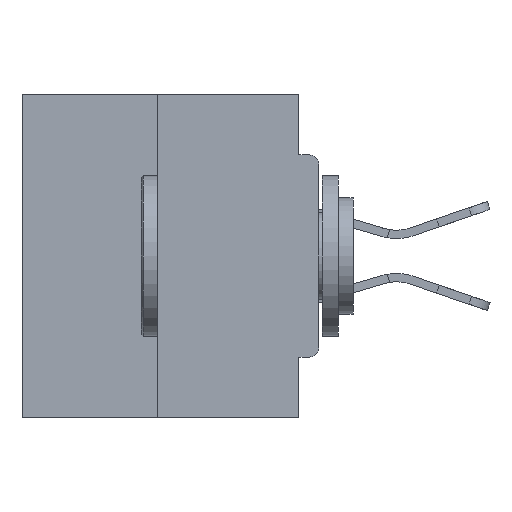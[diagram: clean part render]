
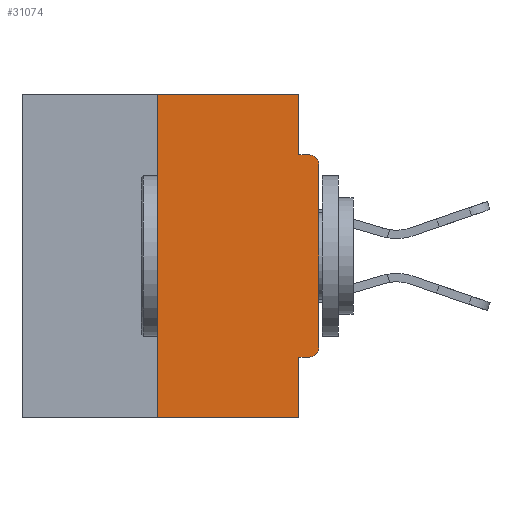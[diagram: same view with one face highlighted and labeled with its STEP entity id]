
A CAD part, left-side view. The second image highlights one B-rep face of the part: STEP entity #31074.
In plain terms, the highlighted planar face has unit normal (-1, 0, 0).
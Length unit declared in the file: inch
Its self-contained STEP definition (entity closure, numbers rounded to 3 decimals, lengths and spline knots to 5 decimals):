
#179 = CARTESIAN_POINT ( 'NONE',  ( 0., 0.25, 0. ) ) ;
#206 = CARTESIAN_POINT ( 'NONE',  ( 0., 0.46, 0. ) ) ;
#354 = VECTOR ( 'NONE', #16216, 39.37008 ) ;
#511 = VECTOR ( 'NONE', #19148, 39.37008 ) ;
#738 = AXIS2_PLACEMENT_3D ( 'NONE', #16466, #16011, #10956 ) ;
#1168 = VERTEX_POINT ( 'NONE', #29994 ) ;
#1659 = CIRCLE ( 'NONE', #30910, 0.015 ) ;
#1946 = CARTESIAN_POINT ( 'NONE',  ( 0., 0.031, 0. ) ) ;
#2277 = ORIENTED_EDGE ( 'NONE', *, *, #3938, .F. ) ;
#2723 = CARTESIAN_POINT ( 'NONE',  ( 0., 0.015, -0.0935 ) ) ;
#3280 = EDGE_CURVE ( 'NONE', #1168, #25429, #1659, .T. ) ;
#3938 = EDGE_CURVE ( 'NONE', #28312, #7588, #29198, .T. ) ;
#5595 = CARTESIAN_POINT ( 'NONE',  ( 0., 0.031, -0.0935 ) ) ;
#6081 = CARTESIAN_POINT ( 'NONE',  ( 0., 0., 0. ) ) ;
#6090 = CARTESIAN_POINT ( 'NONE',  ( 0., 0., -0.3915 ) ) ;
#6240 = VECTOR ( 'NONE', #16872, 39.37008 ) ;
#6244 = EDGE_CURVE ( 'NONE', #25429, #11616, #7592, .T. ) ;
#6886 = DIRECTION ( 'NONE',  ( 0., -1., 0. ) ) ;
#6990 = DIRECTION ( 'NONE',  ( 1., 0., 0. ) ) ;
#7049 = LINE ( 'NONE', #22115, #6240 ) ;
#7381 = CARTESIAN_POINT ( 'NONE',  ( 0., 0.46, -0.5 ) ) ;
#7588 = VERTEX_POINT ( 'NONE', #19410 ) ;
#7592 = LINE ( 'NONE', #6081, #511 ) ;
#8652 = AXIS2_PLACEMENT_3D ( 'NONE', #33786, #6990, #25566 ) ;
#9234 = VECTOR ( 'NONE', #6886, 39.37008 ) ;
#10273 = ORIENTED_EDGE ( 'NONE', *, *, #6244, .T. ) ;
#10285 = CARTESIAN_POINT ( 'NONE',  ( 0., 0.031, -0.5 ) ) ;
#10792 = DIRECTION ( 'NONE',  ( 0., 0., 1. ) ) ;
#10956 = DIRECTION ( 'NONE',  ( 0., 0., -1. ) ) ;
#11283 = LINE ( 'NONE', #7381, #29266 ) ;
#11456 = CARTESIAN_POINT ( 'NONE',  ( 0., 0.031, -0.4065 ) ) ;
#11616 = VERTEX_POINT ( 'NONE', #18738 ) ;
#11720 = ORIENTED_EDGE ( 'NONE', *, *, #3280, .T. ) ;
#12069 = CARTESIAN_POINT ( 'NONE',  ( 0., 0.25, -0.5 ) ) ;
#12322 = VECTOR ( 'NONE', #23061, 39.37008 ) ;
#12788 = DIRECTION ( 'NONE',  ( 0., 1., 0. ) ) ;
#13453 = CARTESIAN_POINT ( 'NONE',  ( 0., 0.015, -0.3915 ) ) ;
#13629 = VERTEX_POINT ( 'NONE', #2723 ) ;
#13695 = DIRECTION ( 'NONE',  ( 0., 0., -1. ) ) ;
#13709 = ORIENTED_EDGE ( 'NONE', *, *, #25088, .F. ) ;
#16011 = DIRECTION ( 'NONE',  ( -1., 0., 0. ) ) ;
#16216 = DIRECTION ( 'NONE',  ( 0., -1., 0. ) ) ;
#16372 = LINE ( 'NONE', #33573, #9234 ) ;
#16466 = CARTESIAN_POINT ( 'NONE',  ( 0., 0.015, -0.1085 ) ) ;
#16708 = EDGE_CURVE ( 'NONE', #1168, #32036, #33486, .T. ) ;
#16737 = ORIENTED_EDGE ( 'NONE', *, *, #19901, .F. ) ;
#16872 = DIRECTION ( 'NONE',  ( 0., 0., -1. ) ) ;
#16969 = EDGE_CURVE ( 'NONE', #32036, #25229, #7049, .T. ) ;
#17366 = ORIENTED_EDGE ( 'NONE', *, *, #26324, .T. ) ;
#17911 = CARTESIAN_POINT ( 'NONE',  ( 0., 0., -0.4065 ) ) ;
#18673 = DIRECTION ( 'NONE',  ( -1., 0., 0. ) ) ;
#18738 = CARTESIAN_POINT ( 'NONE',  ( 0., 0., -0.1085 ) ) ;
#19148 = DIRECTION ( 'NONE',  ( 0., 0., 1. ) ) ;
#19262 = PLANE ( 'NONE',  #8652 ) ;
#19410 = CARTESIAN_POINT ( 'NONE',  ( 0., 0.031, 0. ) ) ;
#19901 = EDGE_CURVE ( 'NONE', #22623, #13629, #16372, .T. ) ;
#21442 = ORIENTED_EDGE ( 'NONE', *, *, #16708, .F. ) ;
#22115 = CARTESIAN_POINT ( 'NONE',  ( 0., 0.031, -0.5 ) ) ;
#22623 = VERTEX_POINT ( 'NONE', #5595 ) ;
#22775 = LINE ( 'NONE', #1946, #12322 ) ;
#23061 = DIRECTION ( 'NONE',  ( 0., 0., -1. ) ) ;
#23544 = CIRCLE ( 'NONE', #738, 0.015 ) ;
#25088 = EDGE_CURVE ( 'NONE', #7588, #22623, #22775, .T. ) ;
#25229 = VERTEX_POINT ( 'NONE', #10285 ) ;
#25429 = VERTEX_POINT ( 'NONE', #6090 ) ;
#25566 = DIRECTION ( 'NONE',  ( 0., 0., -1. ) ) ;
#25662 = CARTESIAN_POINT ( 'NONE',  ( 0., 0.25, 0. ) ) ;
#26110 = ORIENTED_EDGE ( 'NONE', *, *, #16969, .F. ) ;
#26324 = EDGE_CURVE ( 'NONE', #11616, #13629, #23544, .T. ) ;
#26328 = VECTOR ( 'NONE', #12788, 39.37008 ) ;
#27500 = LINE ( 'NONE', #179, #28752 ) ;
#28312 = VERTEX_POINT ( 'NONE', #25662 ) ;
#28752 = VECTOR ( 'NONE', #10792, 39.37008 ) ;
#28952 = VERTEX_POINT ( 'NONE', #12069 ) ;
#29038 = ORIENTED_EDGE ( 'NONE', *, *, #29085, .T. ) ;
#29079 = EDGE_LOOP ( 'NONE', ( #2277, #31316, #29038, #26110, #21442, #11720, #10273, #17366, #16737, #13709 ) ) ;
#29085 = EDGE_CURVE ( 'NONE', #28952, #25229, #11283, .T. ) ;
#29198 = LINE ( 'NONE', #206, #354 ) ;
#29266 = VECTOR ( 'NONE', #31842, 39.37008 ) ;
#29994 = CARTESIAN_POINT ( 'NONE',  ( 0., 0.015, -0.4065 ) ) ;
#30214 = EDGE_CURVE ( 'NONE', #28952, #28312, #27500, .T. ) ;
#30910 = AXIS2_PLACEMENT_3D ( 'NONE', #13453, #18673, #13695 ) ;
#31074 = ADVANCED_FACE ( 'NONE', ( #34598 ), #19262, .F. ) ;
#31316 = ORIENTED_EDGE ( 'NONE', *, *, #30214, .F. ) ;
#31842 = DIRECTION ( 'NONE',  ( 0., -1., 0. ) ) ;
#32036 = VERTEX_POINT ( 'NONE', #11456 ) ;
#33486 = LINE ( 'NONE', #17911, #26328 ) ;
#33573 = CARTESIAN_POINT ( 'NONE',  ( 0., 0., -0.0935 ) ) ;
#33786 = CARTESIAN_POINT ( 'NONE',  ( 0., 0.46, 0. ) ) ;
#34598 = FACE_OUTER_BOUND ( 'NONE', #29079, .T. ) ;
